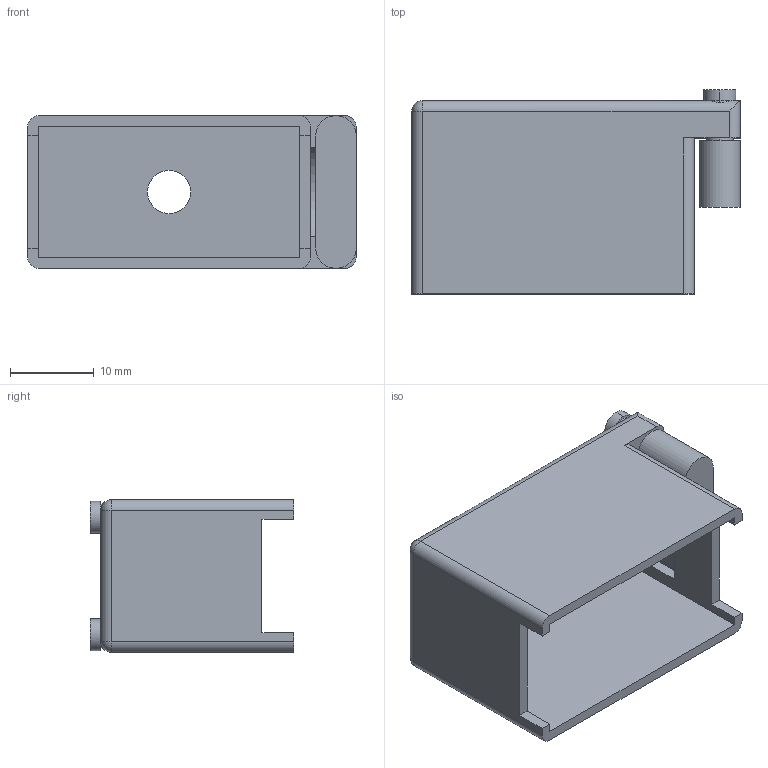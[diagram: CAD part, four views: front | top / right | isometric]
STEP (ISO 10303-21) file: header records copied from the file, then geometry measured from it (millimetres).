
FILE_DESCRIPTION (( 'STEP AP214' ), '1' );
FILE_NAME ('516-230-520.STEP', '2020-08-14T15:30:49', ( '' ), ( '' ), 'SwSTEP 2.0', 'SolidWorks 2020', '' );
FILE_SCHEMA (( 'AUTOMOTIVE_DESIGN' ));
Length unit declared in the file: millimetre
Products named in the file (2): 516-230-520; 516-230-001_Metal - 020 Side Entry
Assembly tree (1 placements, depth 2):
  516-230-520
    516-230-001_Metal - 020 Side Entry
Bounding box: 39.12 x 24.28 x 18.16 mm (x, y, z)
Volume: 3838.9 mm3; surface area: 5816.6 mm2
Topology: 1 solids, 1 shells, 66 faces, 181 edges, 114 vertices
Faces by surface type: plane 35, cylinder 29, sphere 2
Entity records: 2243 total; most frequent: CARTESIAN_POINT 400, DIRECTION 373, ORIENTED_EDGE 358, EDGE_CURVE 179, AXIS2_PLACEMENT_3D 129, LINE 115, VECTOR 115, VERTEX_POINT 114
